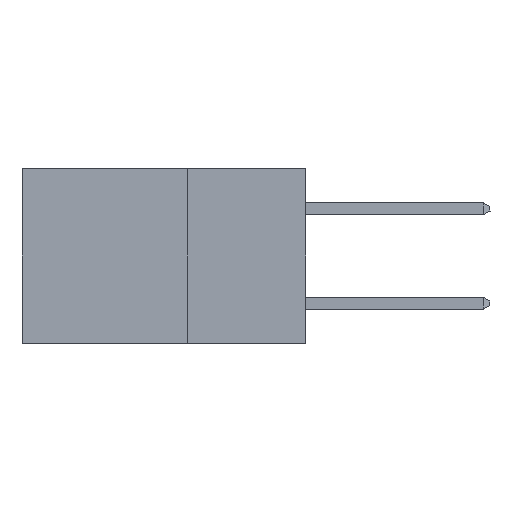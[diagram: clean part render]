
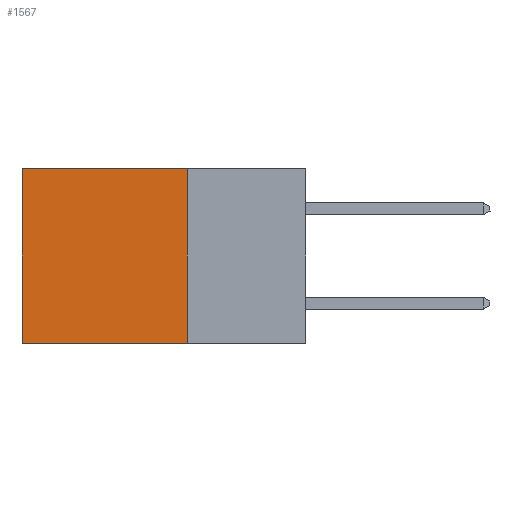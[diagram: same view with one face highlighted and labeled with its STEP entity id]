
A CAD part, left-side view. The second image highlights one B-rep face of the part: STEP entity #1567.
In plain terms, the highlighted planar face has unit normal (-1, 0, 0).
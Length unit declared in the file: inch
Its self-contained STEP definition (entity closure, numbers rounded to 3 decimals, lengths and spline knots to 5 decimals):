
#142 = CARTESIAN_POINT ( 'NONE',  ( 0.298, 0.25, -0.37 ) ) ;
#1567 = ADVANCED_FACE ( 'NONE', ( #7604 ), #9137, .F. ) ;
#1922 = DIRECTION ( 'NONE',  ( 0., 0., -1. ) ) ;
#1977 = CARTESIAN_POINT ( 'NONE',  ( 0.298, 0.25, 0. ) ) ;
#2245 = LINE ( 'NONE', #1977, #9436 ) ;
#2620 = AXIS2_PLACEMENT_3D ( 'NONE', #7598, #4648, #9634 ) ;
#2986 = VECTOR ( 'NONE', #6568, 39.37008 ) ;
#3097 = LINE ( 'NONE', #7643, #8010 ) ;
#3496 = VERTEX_POINT ( 'NONE', #142 ) ;
#3929 = ORIENTED_EDGE ( 'NONE', *, *, #6192, .F. ) ;
#4360 = CARTESIAN_POINT ( 'NONE',  ( 0.298, 0.6, -0.37 ) ) ;
#4522 = DIRECTION ( 'NONE',  ( 0., 0., -1. ) ) ;
#4648 = DIRECTION ( 'NONE',  ( 1., 0., 0. ) ) ;
#4677 = CARTESIAN_POINT ( 'NONE',  ( 0.298, 0.25, -0.37 ) ) ;
#5708 = LINE ( 'NONE', #4677, #2986 ) ;
#6011 = DIRECTION ( 'NONE',  ( 0., 1., 0. ) ) ;
#6152 = ORIENTED_EDGE ( 'NONE', *, *, #11281, .T. ) ;
#6192 = EDGE_CURVE ( 'NONE', #3496, #6340, #5708, .T. ) ;
#6267 = VECTOR ( 'NONE', #1922, 39.37008 ) ;
#6269 = VERTEX_POINT ( 'NONE', #11601 ) ;
#6340 = VERTEX_POINT ( 'NONE', #4360 ) ;
#6568 = DIRECTION ( 'NONE',  ( 0., 1., 0. ) ) ;
#6881 = ORIENTED_EDGE ( 'NONE', *, *, #7977, .F. ) ;
#6975 = CARTESIAN_POINT ( 'NONE',  ( 0.298, 0.25, 0. ) ) ;
#7598 = CARTESIAN_POINT ( 'NONE',  ( 0.298, 0.25, 0. ) ) ;
#7604 = FACE_OUTER_BOUND ( 'NONE', #8670, .T. ) ;
#7643 = CARTESIAN_POINT ( 'NONE',  ( 0.298, 0.25, 0. ) ) ;
#7977 = EDGE_CURVE ( 'NONE', #9336, #3496, #3097, .T. ) ;
#8010 = VECTOR ( 'NONE', #4522, 39.37008 ) ;
#8030 = CARTESIAN_POINT ( 'NONE',  ( 0.298, 0.6, 0. ) ) ;
#8095 = ORIENTED_EDGE ( 'NONE', *, *, #10752, .T. ) ;
#8670 = EDGE_LOOP ( 'NONE', ( #8095, #3929, #6881, #6152 ) ) ;
#9137 = PLANE ( 'NONE',  #2620 ) ;
#9336 = VERTEX_POINT ( 'NONE', #6975 ) ;
#9436 = VECTOR ( 'NONE', #6011, 39.37008 ) ;
#9634 = DIRECTION ( 'NONE',  ( 0., 0., -1. ) ) ;
#10752 = EDGE_CURVE ( 'NONE', #6269, #6340, #11336, .T. ) ;
#11281 = EDGE_CURVE ( 'NONE', #9336, #6269, #2245, .T. ) ;
#11336 = LINE ( 'NONE', #8030, #6267 ) ;
#11601 = CARTESIAN_POINT ( 'NONE',  ( 0.298, 0.6, 0. ) ) ;
